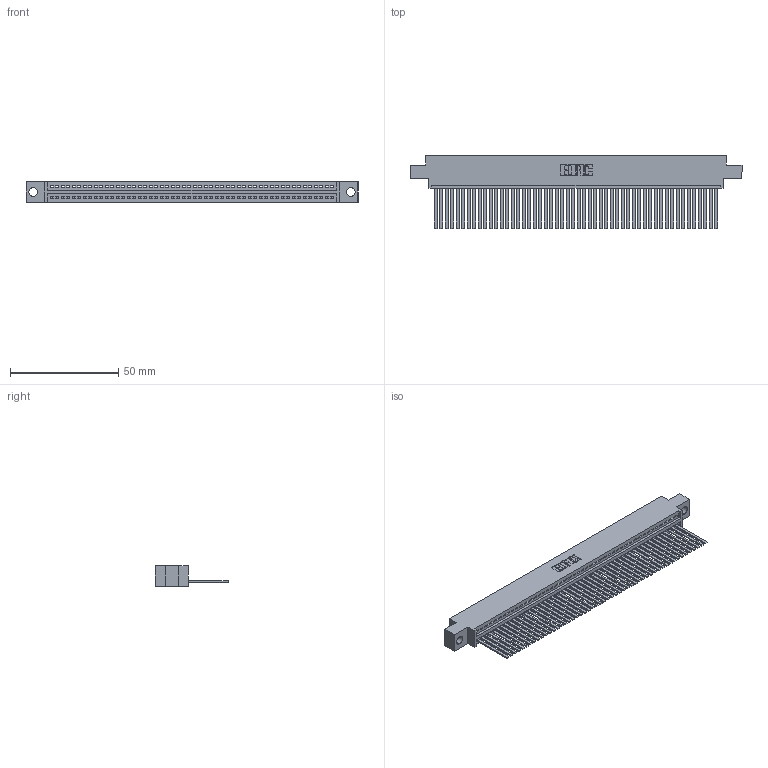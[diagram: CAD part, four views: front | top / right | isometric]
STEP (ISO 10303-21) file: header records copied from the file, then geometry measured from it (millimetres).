
FILE_DESCRIPTION (( 'STEP AP203' ), '1' );
FILE_NAME ('345-052-544-604.STEP', '2018-09-22T23:32:05', ( '' ), ( '' ), 'SwSTEP 2.0', 'SolidWorks 2016', '' );
FILE_SCHEMA (( 'CONFIG_CONTROL_DESIGN' ));
Length unit declared in the file: inch
Products named in the file (3): 345 Part_0.170 Offset - 0.156 Dia-TH; 345-292-001_345-293-144; 345-052-544-604
Assembly tree (53 placements, depth 2):
  345-052-544-604
    345 Part_0.170 Offset - 0.156 Dia-TH
    345-292-001_345-293-144  x52
Bounding box: 153.29 x 33.96 x 9.4 mm (x, y, z)
Volume: 15042.4 mm3; surface area: 21869.2 mm2
Topology: 53 solids, 53 shells, 2834 faces, 8569 edges, 5642 vertices
Faces by surface type: plane 1956, cylinder 878
Entity records: 37741 total; most frequent: CARTESIAN_POINT 6544, ORIENTED_EDGE 6530, DIRECTION 5697, EDGE_CURVE 3265, LINE 2929, VECTOR 2929, VERTEX_POINT 2174, AXIS2_PLACEMENT_3D 1384
